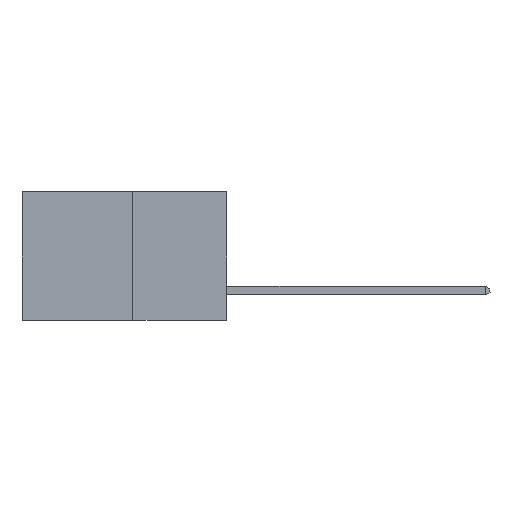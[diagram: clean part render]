
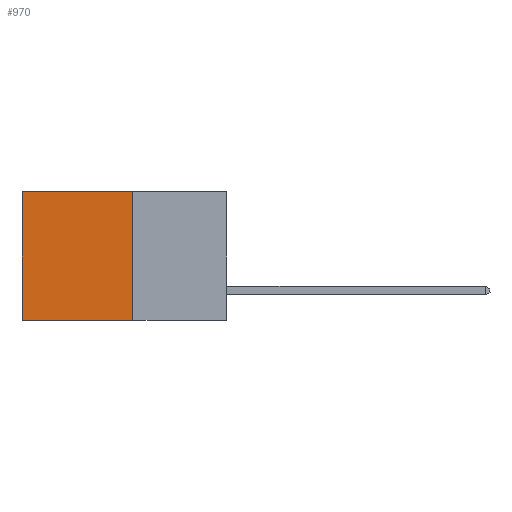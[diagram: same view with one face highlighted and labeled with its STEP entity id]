
A CAD part, left-side view. The second image highlights one B-rep face of the part: STEP entity #970.
In plain terms, the highlighted planar face has unit normal (-1, 0, 0).
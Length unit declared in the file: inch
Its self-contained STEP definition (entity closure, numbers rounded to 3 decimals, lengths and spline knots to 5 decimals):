
#390 = VECTOR ( 'NONE', #9431, 39.37008 ) ;
#490 = DIRECTION ( 'NONE',  ( 1., 0., 0. ) ) ;
#970 = ADVANCED_FACE ( 'NONE', ( #11752 ), #3768, .F. ) ;
#1046 = ORIENTED_EDGE ( 'NONE', *, *, #1778, .F. ) ;
#1778 = EDGE_CURVE ( 'NONE', #4153, #9215, #7369, .T. ) ;
#1861 = LINE ( 'NONE', #6015, #11372 ) ;
#1865 = ORIENTED_EDGE ( 'NONE', *, *, #6284, .F. ) ;
#3589 = DIRECTION ( 'NONE',  ( 0., 0., -1. ) ) ;
#3680 = LINE ( 'NONE', #12026, #390 ) ;
#3750 = CARTESIAN_POINT ( 'NONE',  ( 0.277, 0.27, -0.37 ) ) ;
#3768 = PLANE ( 'NONE',  #6157 ) ;
#3782 = CARTESIAN_POINT ( 'NONE',  ( 0.277, 0.27, -0.37 ) ) ;
#3816 = CARTESIAN_POINT ( 'NONE',  ( 0.277, 0.27, -0.37 ) ) ;
#3853 = VERTEX_POINT ( 'NONE', #11497 ) ;
#4153 = VERTEX_POINT ( 'NONE', #9373 ) ;
#4981 = EDGE_CURVE ( 'NONE', #4153, #3853, #1861, .T. ) ;
#5265 = CARTESIAN_POINT ( 'NONE',  ( 0.277, 0.59, -0.37 ) ) ;
#5579 = DIRECTION ( 'NONE',  ( 0., 1., 0. ) ) ;
#5589 = CARTESIAN_POINT ( 'NONE',  ( 0.277, 0.27, -0.37 ) ) ;
#5669 = DIRECTION ( 'NONE',  ( 0., 1., 0. ) ) ;
#6015 = CARTESIAN_POINT ( 'NONE',  ( 0.277, 0.27, 0. ) ) ;
#6157 = AXIS2_PLACEMENT_3D ( 'NONE', #3782, #490, #8138 ) ;
#6284 = EDGE_CURVE ( 'NONE', #9215, #11716, #10320, .T. ) ;
#7250 = EDGE_CURVE ( 'NONE', #3853, #11716, #3680, .T. ) ;
#7369 = LINE ( 'NONE', #5589, #9391 ) ;
#7738 = EDGE_LOOP ( 'NONE', ( #9455, #1865, #1046, #8789 ) ) ;
#7999 = VECTOR ( 'NONE', #5669, 39.37008 ) ;
#8138 = DIRECTION ( 'NONE',  ( 0., 0., -1. ) ) ;
#8789 = ORIENTED_EDGE ( 'NONE', *, *, #4981, .T. ) ;
#9215 = VERTEX_POINT ( 'NONE', #3750 ) ;
#9373 = CARTESIAN_POINT ( 'NONE',  ( 0.277, 0.27, 0. ) ) ;
#9391 = VECTOR ( 'NONE', #3589, 39.37008 ) ;
#9431 = DIRECTION ( 'NONE',  ( 0., 0., -1. ) ) ;
#9455 = ORIENTED_EDGE ( 'NONE', *, *, #7250, .T. ) ;
#10320 = LINE ( 'NONE', #3816, #7999 ) ;
#11372 = VECTOR ( 'NONE', #5579, 39.37008 ) ;
#11497 = CARTESIAN_POINT ( 'NONE',  ( 0.277, 0.59, 0. ) ) ;
#11716 = VERTEX_POINT ( 'NONE', #5265 ) ;
#11752 = FACE_OUTER_BOUND ( 'NONE', #7738, .T. ) ;
#12026 = CARTESIAN_POINT ( 'NONE',  ( 0.277, 0.59, -0.37 ) ) ;
